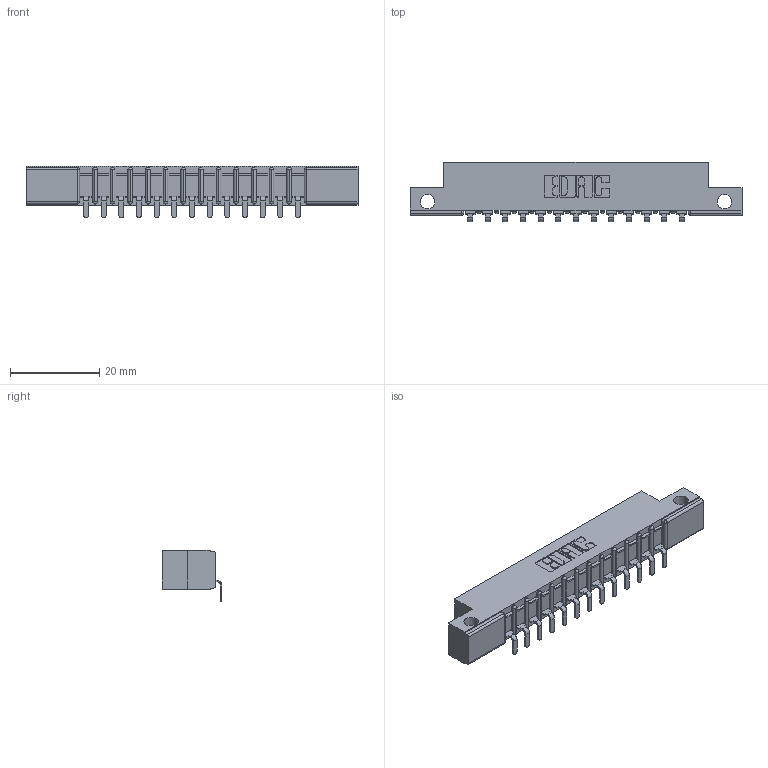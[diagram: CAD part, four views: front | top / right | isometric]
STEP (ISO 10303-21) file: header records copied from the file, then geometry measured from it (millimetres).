
FILE_DESCRIPTION (( 'STEP AP203' ), '1' );
FILE_NAME ('307-013-453-112.STEP', '2020-09-25T14:07:09', ( '' ), ( '' ), 'SwSTEP 2.0', 'SolidWorks 2020', '' );
FILE_SCHEMA (( 'CONFIG_CONTROL_DESIGN' ));
Length unit declared in the file: inch
Products named in the file (7): 307 Part_.128 Dia Side Mounting Holes; 307-013-453-112; 307-290-002_553; #20957; 307-013-454-101; #9888; 307-290-002_554
Assembly tree (14 placements, depth 2):
  307-013-453-112
    307 Part_.128 Dia Side Mounting Holes
    307-290-002_553  x13
  #20957
  307-013-454-101
  #9888
  307-290-002_554
Bounding box: 74.52 x 13.32 x 11.51 mm (x, y, z)
Volume: 4839.2 mm3; surface area: 8167.7 mm2
Topology: 14 solids, 14 shells, 1146 faces, 3495 edges, 2290 vertices
Faces by surface type: plane 681, cylinder 437, sphere 28
Entity records: 34489 total; most frequent: CARTESIAN_POINT 5830, ORIENTED_EDGE 5810, DIRECTION 5666, EDGE_CURVE 2890, VECTOR 2211, LINE 2188, VERTEX_POINT 1865, AXIS2_PLACEMENT_3D 1713
